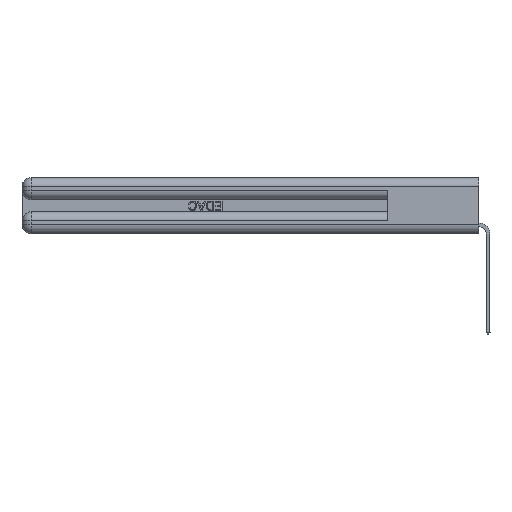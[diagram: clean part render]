
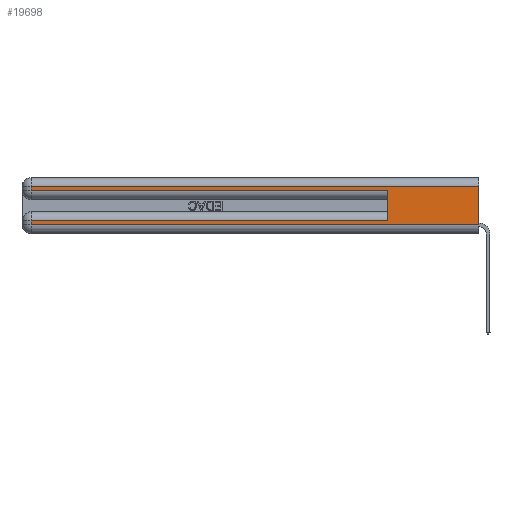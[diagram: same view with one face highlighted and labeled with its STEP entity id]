
A CAD part, left-side view. The second image highlights one B-rep face of the part: STEP entity #19698.
In plain terms, the highlighted planar face has unit normal (-1, 0, 0).
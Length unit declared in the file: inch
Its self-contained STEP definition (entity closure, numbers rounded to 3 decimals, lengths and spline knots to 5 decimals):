
#345 = ORIENTED_EDGE ( 'NONE', *, *, #799, .T. ) ;
#799 = EDGE_CURVE ( 'NONE', #10533, #27249, #7792, .T. ) ;
#901 = LINE ( 'NONE', #17444, #26776 ) ;
#1127 = LINE ( 'NONE', #11609, #9523 ) ;
#1473 = FACE_OUTER_BOUND ( 'NONE', #8007, .T. ) ;
#1505 = EDGE_CURVE ( 'NONE', #10369, #8619, #901, .T. ) ;
#1689 = CARTESIAN_POINT ( 'NONE',  ( 0., 0.6, 0.145 ) ) ;
#1708 = EDGE_CURVE ( 'NONE', #17661, #16523, #14735, .T. ) ;
#2512 = VECTOR ( 'NONE', #16859, 39.37008 ) ;
#2709 = LINE ( 'NONE', #6678, #3364 ) ;
#3009 = ORIENTED_EDGE ( 'NONE', *, *, #6318, .T. ) ;
#3364 = VECTOR ( 'NONE', #7228, 39.37008 ) ;
#3545 = CARTESIAN_POINT ( 'NONE',  ( 0., 2.94, 0.37 ) ) ;
#4023 = CARTESIAN_POINT ( 'NONE',  ( 0., 0., 0.085 ) ) ;
#4395 = EDGE_CURVE ( 'NONE', #10369, #10533, #10238, .T. ) ;
#5232 = ORIENTED_EDGE ( 'NONE', *, *, #5246, .F. ) ;
#5246 = EDGE_CURVE ( 'NONE', #17661, #15457, #6230, .T. ) ;
#5961 = VERTEX_POINT ( 'NONE', #23953 ) ;
#6230 = LINE ( 'NONE', #1689, #17064 ) ;
#6318 = EDGE_CURVE ( 'NONE', #5961, #8619, #2709, .T. ) ;
#6678 = CARTESIAN_POINT ( 'NONE',  ( 0., 0., 0.06 ) ) ;
#7228 = DIRECTION ( 'NONE',  ( 0., -1., 0. ) ) ;
#7430 = CARTESIAN_POINT ( 'NONE',  ( 0., 0., 0.37 ) ) ;
#7509 = DIRECTION ( 'NONE',  ( 0., 0., -1. ) ) ;
#7792 = LINE ( 'NONE', #3545, #22241 ) ;
#7985 = DIRECTION ( 'NONE',  ( 0., 1., 0. ) ) ;
#8007 = EDGE_LOOP ( 'NONE', ( #9998, #24768, #345, #19230, #5232, #25472, #19824, #3009 ) ) ;
#8487 = DIRECTION ( 'NONE',  ( 0., 0., 1. ) ) ;
#8619 = VERTEX_POINT ( 'NONE', #20317 ) ;
#8934 = CARTESIAN_POINT ( 'NONE',  ( 0., 2.94, 0.285 ) ) ;
#9428 = AXIS2_PLACEMENT_3D ( 'NONE', #7430, #22929, #16586 ) ;
#9523 = VECTOR ( 'NONE', #13583, 39.37008 ) ;
#9998 = ORIENTED_EDGE ( 'NONE', *, *, #1505, .F. ) ;
#10238 = LINE ( 'NONE', #16581, #11899 ) ;
#10369 = VERTEX_POINT ( 'NONE', #26888 ) ;
#10393 = DIRECTION ( 'NONE',  ( 0., -1., 0. ) ) ;
#10533 = VERTEX_POINT ( 'NONE', #23664 ) ;
#11609 = CARTESIAN_POINT ( 'NONE',  ( 0., 2.94, 0.37 ) ) ;
#11794 = CARTESIAN_POINT ( 'NONE',  ( 0., 0.6, 0.085 ) ) ;
#11804 = PLANE ( 'NONE',  #9428 ) ;
#11899 = VECTOR ( 'NONE', #7985, 39.37008 ) ;
#12708 = EDGE_CURVE ( 'NONE', #27249, #15457, #17147, .T. ) ;
#13583 = DIRECTION ( 'NONE',  ( 0., 0., -1. ) ) ;
#13625 = CARTESIAN_POINT ( 'NONE',  ( 0., 0.6, 0.285 ) ) ;
#14735 = LINE ( 'NONE', #4023, #2512 ) ;
#15457 = VERTEX_POINT ( 'NONE', #13625 ) ;
#16523 = VERTEX_POINT ( 'NONE', #25585 ) ;
#16581 = CARTESIAN_POINT ( 'NONE',  ( 0., 0., 0.31 ) ) ;
#16586 = DIRECTION ( 'NONE',  ( 0., 0., -1. ) ) ;
#16859 = DIRECTION ( 'NONE',  ( 0., 1., 0. ) ) ;
#17064 = VECTOR ( 'NONE', #8487, 39.37008 ) ;
#17147 = LINE ( 'NONE', #27568, #20764 ) ;
#17444 = CARTESIAN_POINT ( 'NONE',  ( 0., 0., 0.37 ) ) ;
#17661 = VERTEX_POINT ( 'NONE', #11794 ) ;
#19230 = ORIENTED_EDGE ( 'NONE', *, *, #12708, .T. ) ;
#19698 = ADVANCED_FACE ( 'NONE', ( #1473 ), #11804, .F. ) ;
#19824 = ORIENTED_EDGE ( 'NONE', *, *, #24600, .T. ) ;
#20317 = CARTESIAN_POINT ( 'NONE',  ( 0., 0., 0.06 ) ) ;
#20764 = VECTOR ( 'NONE', #10393, 39.37008 ) ;
#22241 = VECTOR ( 'NONE', #7509, 39.37008 ) ;
#22929 = DIRECTION ( 'NONE',  ( 1., 0., 0. ) ) ;
#23664 = CARTESIAN_POINT ( 'NONE',  ( 0., 2.94, 0.31 ) ) ;
#23953 = CARTESIAN_POINT ( 'NONE',  ( 0., 2.94, 0.06 ) ) ;
#24600 = EDGE_CURVE ( 'NONE', #16523, #5961, #1127, .T. ) ;
#24768 = ORIENTED_EDGE ( 'NONE', *, *, #4395, .T. ) ;
#25472 = ORIENTED_EDGE ( 'NONE', *, *, #1708, .T. ) ;
#25585 = CARTESIAN_POINT ( 'NONE',  ( 0., 2.94, 0.085 ) ) ;
#26037 = DIRECTION ( 'NONE',  ( 0., 0., -1. ) ) ;
#26776 = VECTOR ( 'NONE', #26037, 39.37008 ) ;
#26888 = CARTESIAN_POINT ( 'NONE',  ( 0., 0., 0.31 ) ) ;
#27249 = VERTEX_POINT ( 'NONE', #8934 ) ;
#27568 = CARTESIAN_POINT ( 'NONE',  ( 0., 0., 0.285 ) ) ;
